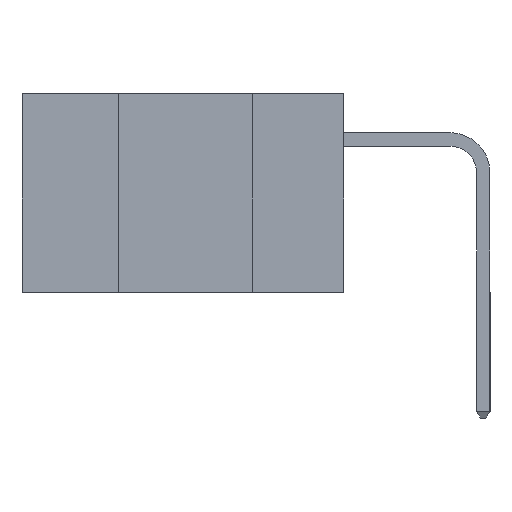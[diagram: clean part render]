
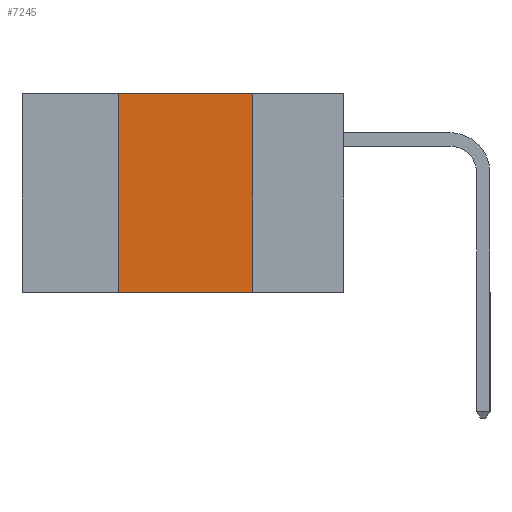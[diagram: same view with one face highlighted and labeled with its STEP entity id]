
A CAD part, left-side view. The second image highlights one B-rep face of the part: STEP entity #7245.
In plain terms, the highlighted planar face has unit normal (-1, 0, 0).
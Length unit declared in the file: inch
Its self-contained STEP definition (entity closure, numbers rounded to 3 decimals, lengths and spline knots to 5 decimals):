
#960 = CARTESIAN_POINT ( 'NONE',  ( 0., 0.17, 0. ) ) ;
#1115 = ORIENTED_EDGE ( 'NONE', *, *, #24580, .F. ) ;
#1346 = LINE ( 'NONE', #9483, #11550 ) ;
#2188 = DIRECTION ( 'NONE',  ( 0., 0., -1. ) ) ;
#2998 = DIRECTION ( 'NONE',  ( 0., 0., -1. ) ) ;
#3298 = LINE ( 'NONE', #960, #23813 ) ;
#3744 = EDGE_CURVE ( 'NONE', #25295, #4407, #13669, .T. ) ;
#3896 = CARTESIAN_POINT ( 'NONE',  ( 0., 0.6, 0. ) ) ;
#4141 = CARTESIAN_POINT ( 'NONE',  ( 0., 0.6, 0. ) ) ;
#4407 = VERTEX_POINT ( 'NONE', #6337 ) ;
#4490 = CARTESIAN_POINT ( 'NONE',  ( 0., 0.6, -0.37 ) ) ;
#5490 = EDGE_LOOP ( 'NONE', ( #9257, #8180, #1115, #5510 ) ) ;
#5510 = ORIENTED_EDGE ( 'NONE', *, *, #3744, .T. ) ;
#6337 = CARTESIAN_POINT ( 'NONE',  ( 0., 0.17, -0.37 ) ) ;
#6486 = CARTESIAN_POINT ( 'NONE',  ( 0., 0.42, 0. ) ) ;
#7245 = ADVANCED_FACE ( 'NONE', ( #21403 ), #12352, .F. ) ;
#7501 = LINE ( 'NONE', #3896, #13565 ) ;
#8180 = ORIENTED_EDGE ( 'NONE', *, *, #21890, .F. ) ;
#8202 = VERTEX_POINT ( 'NONE', #6486 ) ;
#9257 = ORIENTED_EDGE ( 'NONE', *, *, #10960, .F. ) ;
#9483 = CARTESIAN_POINT ( 'NONE',  ( 0., 0.42, 0. ) ) ;
#10960 = EDGE_CURVE ( 'NONE', #21338, #4407, #3298, .T. ) ;
#11550 = VECTOR ( 'NONE', #19824, 39.37008 ) ;
#12352 = PLANE ( 'NONE',  #13109 ) ;
#13109 = AXIS2_PLACEMENT_3D ( 'NONE', #4141, #14416, #2188 ) ;
#13565 = VECTOR ( 'NONE', #16142, 39.37008 ) ;
#13669 = LINE ( 'NONE', #4490, #18508 ) ;
#14416 = DIRECTION ( 'NONE',  ( 1., 0., 0. ) ) ;
#14677 = DIRECTION ( 'NONE',  ( 0., -1., 0. ) ) ;
#16142 = DIRECTION ( 'NONE',  ( 0., -1., 0. ) ) ;
#18508 = VECTOR ( 'NONE', #14677, 39.37008 ) ;
#19824 = DIRECTION ( 'NONE',  ( 0., 0., 1. ) ) ;
#19970 = CARTESIAN_POINT ( 'NONE',  ( 0., 0.42, -0.37 ) ) ;
#21338 = VERTEX_POINT ( 'NONE', #22674 ) ;
#21403 = FACE_OUTER_BOUND ( 'NONE', #5490, .T. ) ;
#21890 = EDGE_CURVE ( 'NONE', #8202, #21338, #7501, .T. ) ;
#22674 = CARTESIAN_POINT ( 'NONE',  ( 0., 0.17, 0. ) ) ;
#23813 = VECTOR ( 'NONE', #2998, 39.37008 ) ;
#24580 = EDGE_CURVE ( 'NONE', #25295, #8202, #1346, .T. ) ;
#25295 = VERTEX_POINT ( 'NONE', #19970 ) ;
